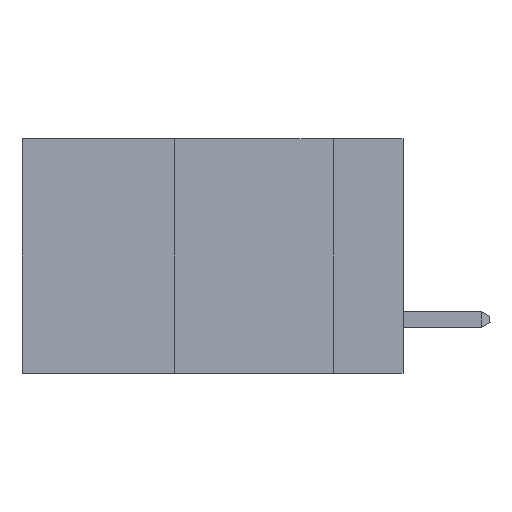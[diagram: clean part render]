
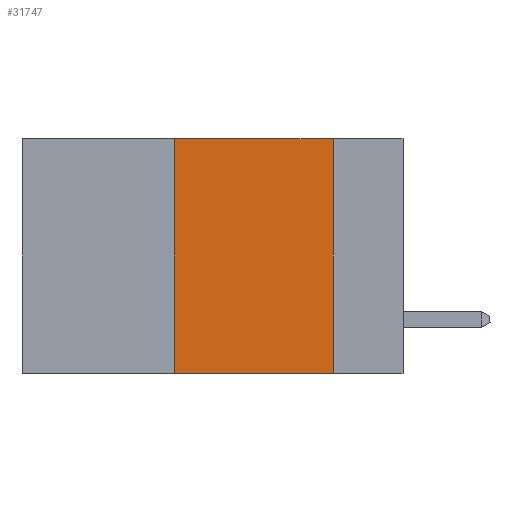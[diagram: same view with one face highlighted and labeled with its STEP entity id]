
A CAD part, left-side view. The second image highlights one B-rep face of the part: STEP entity #31747.
In plain terms, the highlighted planar face has unit normal (-1, 0, 0).
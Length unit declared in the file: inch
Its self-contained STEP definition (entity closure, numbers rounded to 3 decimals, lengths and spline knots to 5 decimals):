
#265 = CARTESIAN_POINT ( 'NONE',  ( 0., 0.11, -0.37 ) ) ;
#1673 = EDGE_CURVE ( 'NONE', #30732, #25158, #29058, .T. ) ;
#2126 = DIRECTION ( 'NONE',  ( 1., 0., 0. ) ) ;
#3122 = DIRECTION ( 'NONE',  ( 0., 0., 1. ) ) ;
#3697 = LINE ( 'NONE', #23544, #24672 ) ;
#5517 = PLANE ( 'NONE',  #32409 ) ;
#5686 = DIRECTION ( 'NONE',  ( 0., -1., 0. ) ) ;
#8497 = VECTOR ( 'NONE', #3122, 39.37008 ) ;
#9213 = FACE_OUTER_BOUND ( 'NONE', #34293, .T. ) ;
#9233 = CARTESIAN_POINT ( 'NONE',  ( 0., 0.36, 0. ) ) ;
#12841 = LINE ( 'NONE', #34240, #8497 ) ;
#14831 = CARTESIAN_POINT ( 'NONE',  ( 0., 0.6, -0.37 ) ) ;
#14864 = EDGE_CURVE ( 'NONE', #23661, #15571, #3697, .T. ) ;
#15115 = CARTESIAN_POINT ( 'NONE',  ( 0., 0.36, -0.37 ) ) ;
#15571 = VERTEX_POINT ( 'NONE', #25909 ) ;
#18078 = ORIENTED_EDGE ( 'NONE', *, *, #14864, .F. ) ;
#20505 = DIRECTION ( 'NONE',  ( 0., -1., 0. ) ) ;
#21740 = VECTOR ( 'NONE', #5686, 39.37008 ) ;
#22701 = VECTOR ( 'NONE', #26787, 39.37008 ) ;
#23544 = CARTESIAN_POINT ( 'NONE',  ( 0., 0.6, 0. ) ) ;
#23661 = VERTEX_POINT ( 'NONE', #9233 ) ;
#23671 = CARTESIAN_POINT ( 'NONE',  ( 0., 0.11, 0. ) ) ;
#24672 = VECTOR ( 'NONE', #20505, 39.37008 ) ;
#25158 = VERTEX_POINT ( 'NONE', #265 ) ;
#25909 = CARTESIAN_POINT ( 'NONE',  ( 0., 0.11, 0. ) ) ;
#26787 = DIRECTION ( 'NONE',  ( 0., 0., -1. ) ) ;
#27323 = DIRECTION ( 'NONE',  ( 0., 0., -1. ) ) ;
#28558 = LINE ( 'NONE', #23671, #22701 ) ;
#29058 = LINE ( 'NONE', #14831, #21740 ) ;
#30732 = VERTEX_POINT ( 'NONE', #15115 ) ;
#31747 = ADVANCED_FACE ( 'NONE', ( #9213 ), #5517, .F. ) ;
#32201 = ORIENTED_EDGE ( 'NONE', *, *, #34464, .F. ) ;
#32409 = AXIS2_PLACEMENT_3D ( 'NONE', #33366, #2126, #27323 ) ;
#32483 = ORIENTED_EDGE ( 'NONE', *, *, #1673, .T. ) ;
#32628 = ORIENTED_EDGE ( 'NONE', *, *, #35408, .F. ) ;
#33366 = CARTESIAN_POINT ( 'NONE',  ( 0., 0.6, 0. ) ) ;
#34240 = CARTESIAN_POINT ( 'NONE',  ( 0., 0.36, 0. ) ) ;
#34293 = EDGE_LOOP ( 'NONE', ( #32201, #18078, #32628, #32483 ) ) ;
#34464 = EDGE_CURVE ( 'NONE', #15571, #25158, #28558, .T. ) ;
#35408 = EDGE_CURVE ( 'NONE', #30732, #23661, #12841, .T. ) ;
